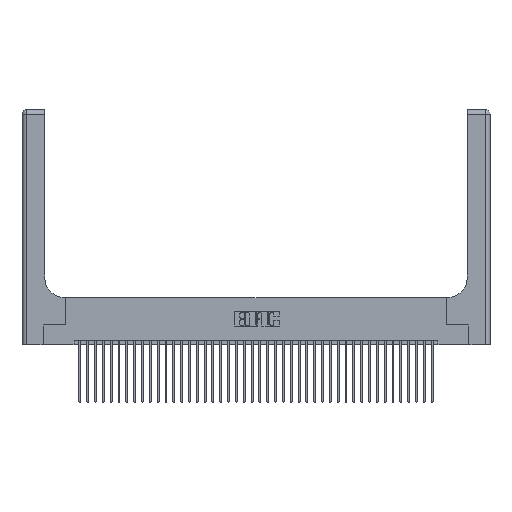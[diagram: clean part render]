
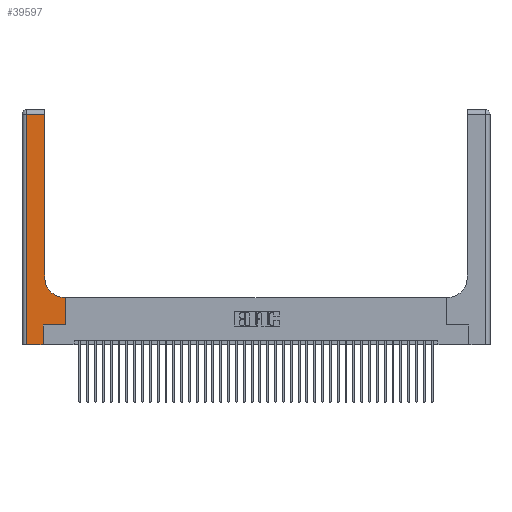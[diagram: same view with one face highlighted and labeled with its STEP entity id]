
A CAD part, top view. The second image highlights one B-rep face of the part: STEP entity #39597.
In plain terms, the highlighted planar face has unit normal (0, 0, 1).
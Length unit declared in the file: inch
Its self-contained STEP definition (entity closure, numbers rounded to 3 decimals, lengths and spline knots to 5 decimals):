
#656 = DIRECTION ( 'NONE',  ( 0., -1., 0. ) ) ;
#1042 = VERTEX_POINT ( 'NONE', #28115 ) ;
#1088 = LINE ( 'NONE', #35727, #13866 ) ;
#1885 = ORIENTED_EDGE ( 'NONE', *, *, #25455, .T. ) ;
#2301 = EDGE_CURVE ( 'NONE', #4504, #2900, #6707, .T. ) ;
#2530 = CARTESIAN_POINT ( 'NONE',  ( 0.269, 0., 0.37 ) ) ;
#2900 = VERTEX_POINT ( 'NONE', #10817 ) ;
#2978 = AXIS2_PLACEMENT_3D ( 'NONE', #12297, #12427, #6385 ) ;
#4504 = VERTEX_POINT ( 'NONE', #38864 ) ;
#5986 = ORIENTED_EDGE ( 'NONE', *, *, #22275, .T. ) ;
#6333 = VECTOR ( 'NONE', #27575, 39.37008 ) ;
#6385 = DIRECTION ( 'NONE',  ( 1., 0., 0. ) ) ;
#6707 = LINE ( 'NONE', #11766, #40771 ) ;
#7007 = EDGE_LOOP ( 'NONE', ( #1885, #5986, #33015, #23740, #31756, #31142, #25904, #13371, #18298 ) ) ;
#7618 = CARTESIAN_POINT ( 'NONE',  ( 0.06, 2.94, 0.37 ) ) ;
#7674 = VERTEX_POINT ( 'NONE', #11300 ) ;
#8050 = VERTEX_POINT ( 'NONE', #16152 ) ;
#8782 = DIRECTION ( 'NONE',  ( 0., 1., 0. ) ) ;
#8916 = LINE ( 'NONE', #11323, #33176 ) ;
#10142 = CARTESIAN_POINT ( 'NONE',  ( 0.5585, 0.6, 0.37 ) ) ;
#10817 = CARTESIAN_POINT ( 'NONE',  ( 0.269, 0., 0.37 ) ) ;
#11300 = CARTESIAN_POINT ( 'NONE',  ( 0.5415, 0.6, 0.37 ) ) ;
#11323 = CARTESIAN_POINT ( 'NONE',  ( 0., 2.94, 0.37 ) ) ;
#11766 = CARTESIAN_POINT ( 'NONE',  ( 0., 0., 0.37 ) ) ;
#12297 = CARTESIAN_POINT ( 'NONE',  ( 0.5415, 0.85, 0.37 ) ) ;
#12427 = DIRECTION ( 'NONE',  ( 0., 0., -1. ) ) ;
#13371 = ORIENTED_EDGE ( 'NONE', *, *, #25689, .T. ) ;
#13866 = VECTOR ( 'NONE', #656, 39.37008 ) ;
#13895 = DIRECTION ( 'NONE',  ( -1., 0., 0. ) ) ;
#14011 = EDGE_CURVE ( 'NONE', #27669, #4504, #1088, .T. ) ;
#14663 = VECTOR ( 'NONE', #13895, 39.37008 ) ;
#15579 = CARTESIAN_POINT ( 'NONE',  ( 0.269, 0.25, 0.37 ) ) ;
#16152 = CARTESIAN_POINT ( 'NONE',  ( 0.2915, 2.94, 0.37 ) ) ;
#16185 = LINE ( 'NONE', #34427, #37424 ) ;
#17175 = LINE ( 'NONE', #29661, #22636 ) ;
#18298 = ORIENTED_EDGE ( 'NONE', *, *, #22486, .T. ) ;
#18871 = CIRCLE ( 'NONE', #2978, 0.25 ) ;
#21791 = VERTEX_POINT ( 'NONE', #15579 ) ;
#22275 = EDGE_CURVE ( 'NONE', #8050, #27669, #8916, .T. ) ;
#22486 = EDGE_CURVE ( 'NONE', #7674, #1042, #18871, .T. ) ;
#22636 = VECTOR ( 'NONE', #35945, 39.37008 ) ;
#23459 = VERTEX_POINT ( 'NONE', #10142 ) ;
#23740 = ORIENTED_EDGE ( 'NONE', *, *, #2301, .T. ) ;
#24564 = DIRECTION ( 'NONE',  ( 1., 0., 0. ) ) ;
#25455 = EDGE_CURVE ( 'NONE', #1042, #8050, #16185, .T. ) ;
#25689 = EDGE_CURVE ( 'NONE', #23459, #7674, #31535, .T. ) ;
#25904 = ORIENTED_EDGE ( 'NONE', *, *, #39335, .T. ) ;
#26126 = LINE ( 'NONE', #2530, #39872 ) ;
#26570 = PLANE ( 'NONE',  #38232 ) ;
#27575 = DIRECTION ( 'NONE',  ( 0., 1., 0. ) ) ;
#27669 = VERTEX_POINT ( 'NONE', #7618 ) ;
#28115 = CARTESIAN_POINT ( 'NONE',  ( 0.2915, 0.85, 0.37 ) ) ;
#29661 = CARTESIAN_POINT ( 'NONE',  ( 0.269, 0.25, 0.37 ) ) ;
#31142 = ORIENTED_EDGE ( 'NONE', *, *, #39214, .T. ) ;
#31535 = LINE ( 'NONE', #39028, #14663 ) ;
#31580 = EDGE_CURVE ( 'NONE', #2900, #21791, #26126, .T. ) ;
#31756 = ORIENTED_EDGE ( 'NONE', *, *, #31580, .T. ) ;
#31812 = DIRECTION ( 'NONE',  ( 0., 1., 0. ) ) ;
#32372 = DIRECTION ( 'NONE',  ( 0., 0., -1. ) ) ;
#32546 = LINE ( 'NONE', #39742, #6333 ) ;
#32918 = CARTESIAN_POINT ( 'NONE',  ( 0., 3., 0.37 ) ) ;
#33015 = ORIENTED_EDGE ( 'NONE', *, *, #14011, .T. ) ;
#33176 = VECTOR ( 'NONE', #36214, 39.37008 ) ;
#34427 = CARTESIAN_POINT ( 'NONE',  ( 0.2915, 3., 0.37 ) ) ;
#35442 = FACE_OUTER_BOUND ( 'NONE', #7007, .T. ) ;
#35727 = CARTESIAN_POINT ( 'NONE',  ( 0.06, 3., 0.37 ) ) ;
#35945 = DIRECTION ( 'NONE',  ( 1., 0., 0. ) ) ;
#36214 = DIRECTION ( 'NONE',  ( -1., 0., 0. ) ) ;
#36229 = VERTEX_POINT ( 'NONE', #37387 ) ;
#37387 = CARTESIAN_POINT ( 'NONE',  ( 0.5585, 0.25, 0.37 ) ) ;
#37424 = VECTOR ( 'NONE', #31812, 39.37008 ) ;
#38232 = AXIS2_PLACEMENT_3D ( 'NONE', #32918, #32372, #38522 ) ;
#38522 = DIRECTION ( 'NONE',  ( -1., 0., 0. ) ) ;
#38864 = CARTESIAN_POINT ( 'NONE',  ( 0.06, 0., 0.37 ) ) ;
#39028 = CARTESIAN_POINT ( 'NONE',  ( 0.2915, 0.6, 0.37 ) ) ;
#39214 = EDGE_CURVE ( 'NONE', #21791, #36229, #17175, .T. ) ;
#39335 = EDGE_CURVE ( 'NONE', #36229, #23459, #32546, .T. ) ;
#39597 = ADVANCED_FACE ( 'NONE', ( #35442 ), #26570, .F. ) ;
#39742 = CARTESIAN_POINT ( 'NONE',  ( 0.5585, 0.25, 0.37 ) ) ;
#39872 = VECTOR ( 'NONE', #8782, 39.37008 ) ;
#40771 = VECTOR ( 'NONE', #24564, 39.37008 ) ;
